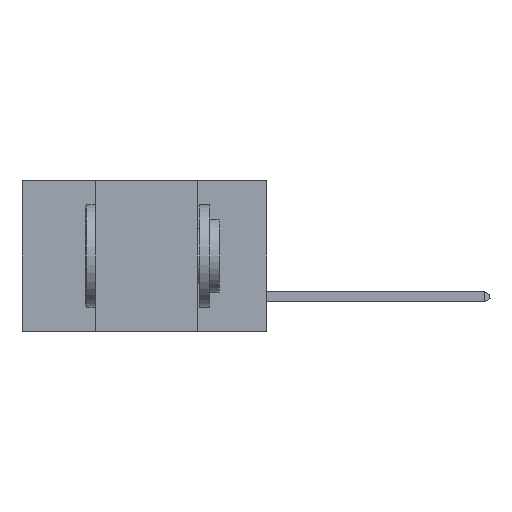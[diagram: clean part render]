
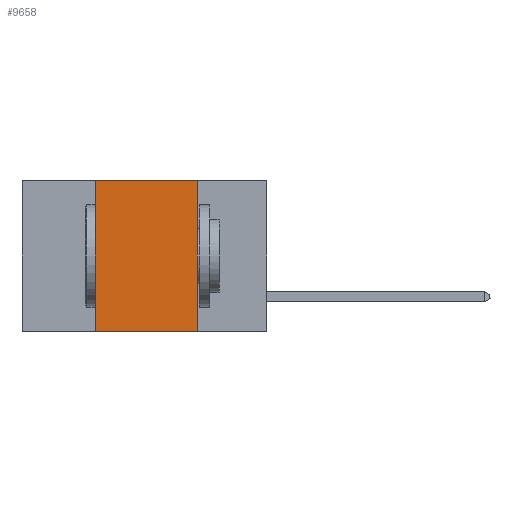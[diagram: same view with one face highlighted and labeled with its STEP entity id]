
A CAD part, left-side view. The second image highlights one B-rep face of the part: STEP entity #9658.
In plain terms, the highlighted planar face has unit normal (-1, 0, 0).
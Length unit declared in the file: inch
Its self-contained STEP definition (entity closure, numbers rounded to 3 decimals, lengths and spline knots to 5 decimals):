
#193 = CARTESIAN_POINT ( 'NONE',  ( 0., 0.17, 0. ) ) ;
#1047 = EDGE_CURVE ( 'NONE', #24424, #9728, #2853, .T. ) ;
#2333 = PLANE ( 'NONE',  #5420 ) ;
#2853 = LINE ( 'NONE', #20898, #11635 ) ;
#4111 = DIRECTION ( 'NONE',  ( 1., 0., 0. ) ) ;
#5420 = AXIS2_PLACEMENT_3D ( 'NONE', #24451, #4111, #8523 ) ;
#6266 = EDGE_CURVE ( 'NONE', #24925, #13305, #12638, .T. ) ;
#7519 = DIRECTION ( 'NONE',  ( 0., -1., 0. ) ) ;
#7558 = EDGE_CURVE ( 'NONE', #24424, #24925, #13190, .T. ) ;
#7753 = CARTESIAN_POINT ( 'NONE',  ( 0., 0.42, 0. ) ) ;
#7813 = VECTOR ( 'NONE', #16279, 39.37008 ) ;
#8523 = DIRECTION ( 'NONE',  ( 0., 0., -1. ) ) ;
#9502 = DIRECTION ( 'NONE',  ( 0., 0., 1. ) ) ;
#9658 = ADVANCED_FACE ( 'NONE', ( #16777 ), #2333, .F. ) ;
#9728 = VERTEX_POINT ( 'NONE', #20332 ) ;
#10738 = CARTESIAN_POINT ( 'NONE',  ( 0., 0.42, -0.37 ) ) ;
#11289 = VECTOR ( 'NONE', #9502, 39.37008 ) ;
#11430 = CARTESIAN_POINT ( 'NONE',  ( 0., 0.42, 0. ) ) ;
#11635 = VECTOR ( 'NONE', #22927, 39.37008 ) ;
#11821 = CARTESIAN_POINT ( 'NONE',  ( 0., 0.17, 0. ) ) ;
#12214 = ORIENTED_EDGE ( 'NONE', *, *, #1047, .T. ) ;
#12638 = LINE ( 'NONE', #19668, #25661 ) ;
#13149 = LINE ( 'NONE', #11821, #7813 ) ;
#13190 = LINE ( 'NONE', #11430, #11289 ) ;
#13305 = VERTEX_POINT ( 'NONE', #193 ) ;
#15313 = ORIENTED_EDGE ( 'NONE', *, *, #25506, .F. ) ;
#15346 = EDGE_LOOP ( 'NONE', ( #15313, #19300, #25441, #12214 ) ) ;
#16279 = DIRECTION ( 'NONE',  ( 0., 0., -1. ) ) ;
#16777 = FACE_OUTER_BOUND ( 'NONE', #15346, .T. ) ;
#19300 = ORIENTED_EDGE ( 'NONE', *, *, #6266, .F. ) ;
#19668 = CARTESIAN_POINT ( 'NONE',  ( 0., 0.6, 0. ) ) ;
#20332 = CARTESIAN_POINT ( 'NONE',  ( 0., 0.17, -0.37 ) ) ;
#20898 = CARTESIAN_POINT ( 'NONE',  ( 0., 0.6, -0.37 ) ) ;
#22927 = DIRECTION ( 'NONE',  ( 0., -1., 0. ) ) ;
#24424 = VERTEX_POINT ( 'NONE', #10738 ) ;
#24451 = CARTESIAN_POINT ( 'NONE',  ( 0., 0.6, 0. ) ) ;
#24925 = VERTEX_POINT ( 'NONE', #7753 ) ;
#25441 = ORIENTED_EDGE ( 'NONE', *, *, #7558, .F. ) ;
#25506 = EDGE_CURVE ( 'NONE', #13305, #9728, #13149, .T. ) ;
#25661 = VECTOR ( 'NONE', #7519, 39.37008 ) ;
